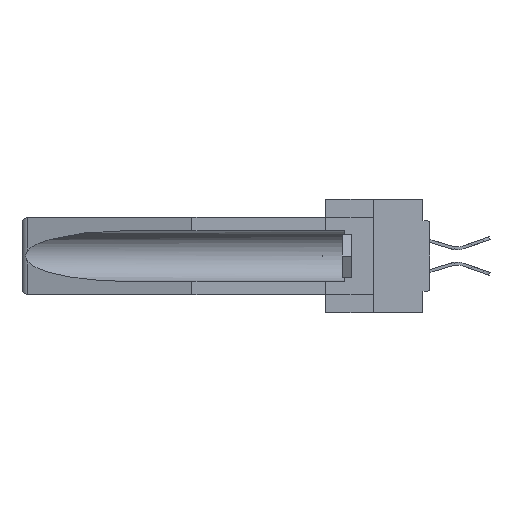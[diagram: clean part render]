
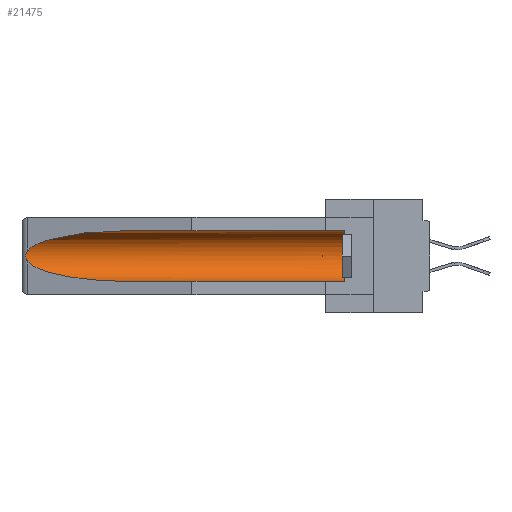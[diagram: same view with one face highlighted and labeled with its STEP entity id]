
A CAD part, left-side view. The second image highlights one B-rep face of the part: STEP entity #21475.
In plain terms, the highlighted cylindrical face has radius 2.857 mm (diameter 5.715 mm), a partial arc.
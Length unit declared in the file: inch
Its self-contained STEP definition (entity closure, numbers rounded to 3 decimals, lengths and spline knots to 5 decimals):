
#187 = CARTESIAN_POINT ( 'NONE',  ( 0.26537, 1.52718, -0.19328 ) ) ;
#350 = CARTESIAN_POINT ( 'NONE',  ( 0.2675, 1.53308, -0.16763 ) ) ;
#437 = EDGE_CURVE ( 'NONE', #11281, #24977, #20880, .T. ) ;
#961 = VECTOR ( 'NONE', #29703, 39.37008 ) ;
#1184 = LINE ( 'NONE', #29363, #32264 ) ;
#2083 = CARTESIAN_POINT ( 'NONE',  ( 0.26537, 1.52718, -0.14972 ) ) ;
#2753 = CARTESIAN_POINT ( 'NONE',  ( 0.21114, 1.30732, -0.059 ) ) ;
#2999 = VERTEX_POINT ( 'NONE', #6929 ) ;
#3549 = CARTESIAN_POINT ( 'NONE',  ( 0.155, -0.30754, -0.059 ) ) ;
#3985 = CARTESIAN_POINT ( 'NONE',  ( 0.26597, 1.52961, -0.15275 ) ) ;
#4300 = CARTESIAN_POINT ( 'NONE',  ( 0.26654, 1.53092, -0.15636 ) ) ;
#5217 =( BOUNDED_CURVE ( )  B_SPLINE_CURVE ( 3, ( #9625, #2753, #32710, #2083 ),
 .UNSPECIFIED., .F., .F. ) 
 B_SPLINE_CURVE_WITH_KNOTS ( ( 4, 4 ),
 ( 4.71239, 6.08839 ),
 .UNSPECIFIED. ) 
 CURVE ( )  GEOMETRIC_REPRESENTATION_ITEM ( )  RATIONAL_B_SPLINE_CURVE ( ( 1., 0.848, 0.848, 1. ) ) 
 REPRESENTATION_ITEM ( '' )  );
#6420 = AXIS2_PLACEMENT_3D ( 'NONE', #7592, #15118, #45118 ) ;
#6929 = CARTESIAN_POINT ( 'NONE',  ( 0.155, 1.07973, -0.284 ) ) ;
#7592 = CARTESIAN_POINT ( 'NONE',  ( 0.155, 0.126, -0.1715 ) ) ;
#7827 = CARTESIAN_POINT ( 'NONE',  ( 0.26537, 1.52718, -0.19328 ) ) ;
#8308 = DIRECTION ( 'NONE',  ( 0., 1., 0. ) ) ;
#9572 = VERTEX_POINT ( 'NONE', #24515 ) ;
#9625 = CARTESIAN_POINT ( 'NONE',  ( 0.155, 1.07973, -0.059 ) ) ;
#9923 = EDGE_CURVE ( 'NONE', #9572, #2999, #1184, .T. ) ;
#10815 = ORIENTED_EDGE ( 'NONE', *, *, #29700, .T. ) ;
#11281 = VERTEX_POINT ( 'NONE', #33602 ) ;
#11435 = CARTESIAN_POINT ( 'NONE',  ( 0.155, 1.07973, -0.284 ) ) ;
#14270 = ORIENTED_EDGE ( 'NONE', *, *, #19688, .T. ) ;
#14927 = CARTESIAN_POINT ( 'NONE',  ( 0.26655, 1.53094, -0.18657 ) ) ;
#15118 = DIRECTION ( 'NONE',  ( 0., -1., 0. ) ) ;
#15591 = FACE_OUTER_BOUND ( 'NONE', #32413, .T. ) ;
#15725 = VERTEX_POINT ( 'NONE', #47318 ) ;
#16183 = ORIENTED_EDGE ( 'NONE', *, *, #9923, .F. ) ;
#17498 =( BOUNDED_CURVE ( )  B_SPLINE_CURVE ( 3, ( #7827, #37790, #26644, #11435 ),
 .UNSPECIFIED., .F., .F. ) 
 B_SPLINE_CURVE_WITH_KNOTS ( ( 4, 4 ),
 ( 0.1948, 1.5708 ),
 .UNSPECIFIED. ) 
 CURVE ( )  GEOMETRIC_REPRESENTATION_ITEM ( )  RATIONAL_B_SPLINE_CURVE ( ( 1., 0.848, 0.848, 1. ) ) 
 REPRESENTATION_ITEM ( '' )  );
#17527 = ORIENTED_EDGE ( 'NONE', *, *, #29561, .T. ) ;
#17850 = ORIENTED_EDGE ( 'NONE', *, *, #47109, .T. ) ;
#19688 = EDGE_CURVE ( 'NONE', #9572, #11281, #37869, .T. ) ;
#20880 = LINE ( 'NONE', #3549, #961 ) ;
#21475 = ADVANCED_FACE ( 'NONE', ( #15591 ), #47901, .F. ) ;
#21814 = CARTESIAN_POINT ( 'NONE',  ( 0.26537, 1.52718, -0.14972 ) ) ;
#24358 = ORIENTED_EDGE ( 'NONE', *, *, #437, .T. ) ;
#24515 = CARTESIAN_POINT ( 'NONE',  ( 0.155, 0.126, -0.284 ) ) ;
#24977 = VERTEX_POINT ( 'NONE', #43044 ) ;
#26206 = B_SPLINE_CURVE_WITH_KNOTS ( 'NONE', 3,
 ( #41495, #3985, #4300, #30466, #350, #48532, #45412, #14927, #26554, #187 ),
 .UNSPECIFIED., .F., .F.,
 ( 4, 2, 2, 2, 4 ),
 ( 0., 0.00029, 0.00058, 0.00087, 0.00117 ),
 .UNSPECIFIED. ) ;
#26554 = CARTESIAN_POINT ( 'NONE',  ( 0.26597, 1.5296, -0.19026 ) ) ;
#26644 = CARTESIAN_POINT ( 'NONE',  ( 0.21114, 1.30732, -0.284 ) ) ;
#29363 = CARTESIAN_POINT ( 'NONE',  ( 0.155, -0.30754, -0.284 ) ) ;
#29561 = EDGE_CURVE ( 'NONE', #43577, #15725, #26206, .T. ) ;
#29700 = EDGE_CURVE ( 'NONE', #24977, #43577, #5217, .T. ) ;
#29703 = DIRECTION ( 'NONE',  ( 0., 1., 0. ) ) ;
#30466 = CARTESIAN_POINT ( 'NONE',  ( 0.2673, 1.5327, -0.16383 ) ) ;
#30879 = DIRECTION ( 'NONE',  ( 0., 0., 1. ) ) ;
#32264 = VECTOR ( 'NONE', #47058, 39.37008 ) ;
#32413 = EDGE_LOOP ( 'NONE', ( #10815, #17527, #17850, #16183, #14270, #24358 ) ) ;
#32710 = CARTESIAN_POINT ( 'NONE',  ( 0.25451, 1.48313, -0.09465 ) ) ;
#33602 = CARTESIAN_POINT ( 'NONE',  ( 0.155, 0.126, -0.059 ) ) ;
#36878 = AXIS2_PLACEMENT_3D ( 'NONE', #45365, #8308, #30879 ) ;
#37790 = CARTESIAN_POINT ( 'NONE',  ( 0.25451, 1.48313, -0.24835 ) ) ;
#37869 = CIRCLE ( 'NONE', #6420, 0.1125 ) ;
#41495 = CARTESIAN_POINT ( 'NONE',  ( 0.26537, 1.52718, -0.14972 ) ) ;
#43044 = CARTESIAN_POINT ( 'NONE',  ( 0.155, 1.07973, -0.059 ) ) ;
#43577 = VERTEX_POINT ( 'NONE', #21814 ) ;
#45118 = DIRECTION ( 'NONE',  ( 0., 0., 1. ) ) ;
#45365 = CARTESIAN_POINT ( 'NONE',  ( 0.155, -0.30754, -0.1715 ) ) ;
#45412 = CARTESIAN_POINT ( 'NONE',  ( 0.2673, 1.53269, -0.17917 ) ) ;
#47058 = DIRECTION ( 'NONE',  ( 0., 1., 0. ) ) ;
#47109 = EDGE_CURVE ( 'NONE', #15725, #2999, #17498, .T. ) ;
#47318 = CARTESIAN_POINT ( 'NONE',  ( 0.26537, 1.52718, -0.19328 ) ) ;
#47901 = CYLINDRICAL_SURFACE ( 'NONE', #36878, 0.1125 ) ;
#48532 = CARTESIAN_POINT ( 'NONE',  ( 0.2675, 1.53308, -0.17534 ) ) ;
